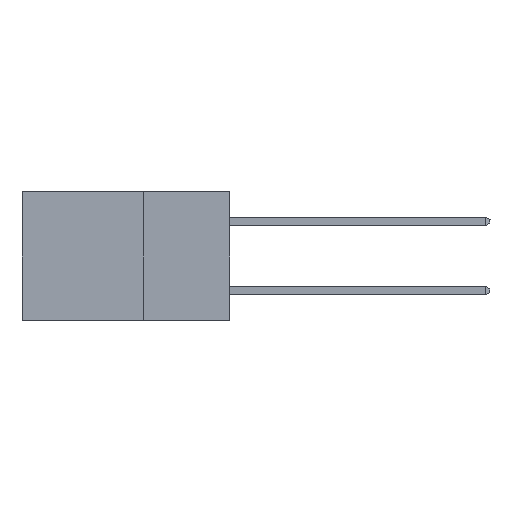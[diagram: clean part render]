
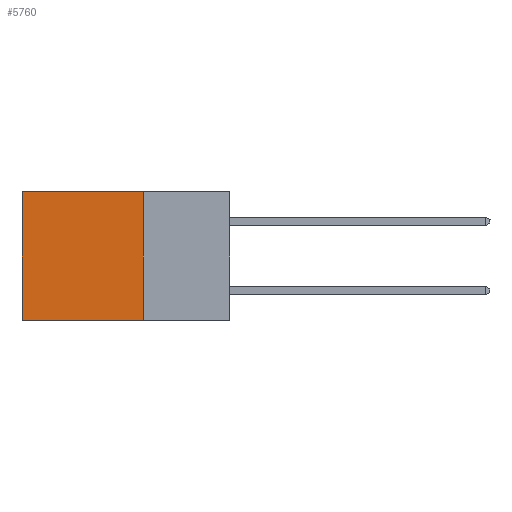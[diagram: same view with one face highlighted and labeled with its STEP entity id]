
A CAD part, left-side view. The second image highlights one B-rep face of the part: STEP entity #5760.
In plain terms, the highlighted planar face has unit normal (-1, 0, 0).
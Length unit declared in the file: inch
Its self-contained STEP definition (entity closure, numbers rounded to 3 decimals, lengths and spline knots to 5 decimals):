
#510 = CARTESIAN_POINT ( 'NONE',  ( 0.2615, 0.25, -0.37 ) ) ;
#544 = VECTOR ( 'NONE', #3830, 39.37008 ) ;
#731 = LINE ( 'NONE', #6881, #544 ) ;
#817 = DIRECTION ( 'NONE',  ( 1., 0., 0. ) ) ;
#1015 = CARTESIAN_POINT ( 'NONE',  ( 0.2615, 0.25, -0.37 ) ) ;
#1033 = CARTESIAN_POINT ( 'NONE',  ( 0.2615, 0.25, 0. ) ) ;
#1052 = VECTOR ( 'NONE', #1316, 39.37008 ) ;
#1316 = DIRECTION ( 'NONE',  ( 0., 1., 0. ) ) ;
#1433 = LINE ( 'NONE', #510, #1052 ) ;
#1803 = CARTESIAN_POINT ( 'NONE',  ( 0.2615, 0.6, -0.37 ) ) ;
#2393 = PLANE ( 'NONE',  #7381 ) ;
#2464 = EDGE_CURVE ( 'NONE', #2981, #5499, #731, .T. ) ;
#2593 = EDGE_LOOP ( 'NONE', ( #9381, #7007, #4754, #9657 ) ) ;
#2598 = DIRECTION ( 'NONE',  ( 0., 1., 0. ) ) ;
#2981 = VERTEX_POINT ( 'NONE', #7161 ) ;
#3830 = DIRECTION ( 'NONE',  ( 0., 0., -1. ) ) ;
#3971 = CARTESIAN_POINT ( 'NONE',  ( 0.2615, 0.25, -0.37 ) ) ;
#4697 = EDGE_CURVE ( 'NONE', #9565, #2981, #8648, .T. ) ;
#4754 = ORIENTED_EDGE ( 'NONE', *, *, #8216, .F. ) ;
#4872 = EDGE_CURVE ( 'NONE', #10024, #5499, #1433, .T. ) ;
#5415 = CARTESIAN_POINT ( 'NONE',  ( 0.2615, 0.25, 0. ) ) ;
#5499 = VERTEX_POINT ( 'NONE', #1803 ) ;
#5760 = ADVANCED_FACE ( 'NONE', ( #7953 ), #2393, .F. ) ;
#6204 = VECTOR ( 'NONE', #9310, 39.37008 ) ;
#6881 = CARTESIAN_POINT ( 'NONE',  ( 0.2615, 0.6, -0.37 ) ) ;
#7007 = ORIENTED_EDGE ( 'NONE', *, *, #4872, .F. ) ;
#7047 = VECTOR ( 'NONE', #2598, 39.37008 ) ;
#7161 = CARTESIAN_POINT ( 'NONE',  ( 0.2615, 0.6, 0. ) ) ;
#7381 = AXIS2_PLACEMENT_3D ( 'NONE', #3971, #817, #7907 ) ;
#7907 = DIRECTION ( 'NONE',  ( 0., 0., -1. ) ) ;
#7953 = FACE_OUTER_BOUND ( 'NONE', #2593, .T. ) ;
#8216 = EDGE_CURVE ( 'NONE', #9565, #10024, #9936, .T. ) ;
#8432 = CARTESIAN_POINT ( 'NONE',  ( 0.2615, 0.25, -0.37 ) ) ;
#8648 = LINE ( 'NONE', #1033, #7047 ) ;
#9310 = DIRECTION ( 'NONE',  ( 0., 0., -1. ) ) ;
#9381 = ORIENTED_EDGE ( 'NONE', *, *, #2464, .T. ) ;
#9565 = VERTEX_POINT ( 'NONE', #5415 ) ;
#9657 = ORIENTED_EDGE ( 'NONE', *, *, #4697, .T. ) ;
#9936 = LINE ( 'NONE', #8432, #6204 ) ;
#10024 = VERTEX_POINT ( 'NONE', #1015 ) ;
